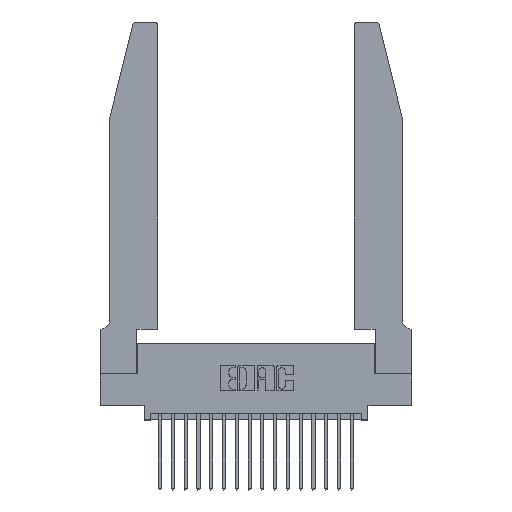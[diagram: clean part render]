
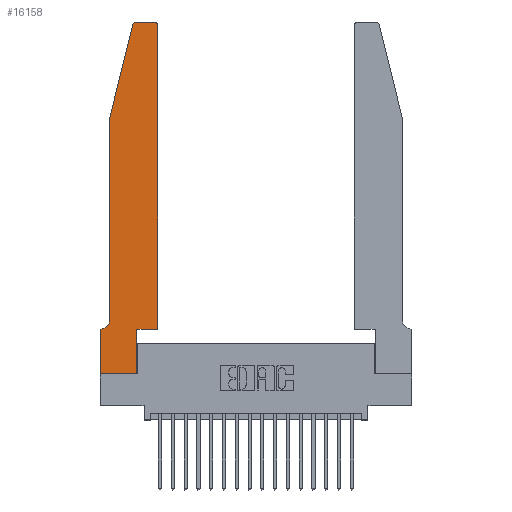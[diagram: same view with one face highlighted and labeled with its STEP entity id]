
A CAD part, top view. The second image highlights one B-rep face of the part: STEP entity #16158.
In plain terms, the highlighted planar face has unit normal (0, 0, 1).
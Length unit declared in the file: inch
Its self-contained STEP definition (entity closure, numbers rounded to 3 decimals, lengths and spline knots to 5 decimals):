
#399 = AXIS2_PLACEMENT_3D ( 'NONE', #18051, #5147, #11506 ) ;
#463 = VERTEX_POINT ( 'NONE', #5191 ) ;
#599 = CARTESIAN_POINT ( 'NONE',  ( 0.4205, 2.75, 0.37 ) ) ;
#695 = CARTESIAN_POINT ( 'NONE',  ( 0.4505, 0.35, 0.37 ) ) ;
#801 = DIRECTION ( 'NONE',  ( 1., 0., 0. ) ) ;
#951 = CARTESIAN_POINT ( 'NONE',  ( 0.0755, 2., 0.37 ) ) ;
#1317 = ORIENTED_EDGE ( 'NONE', *, *, #19890, .T. ) ;
#1614 = DIRECTION ( 'NONE',  ( 0., 0., -1. ) ) ;
#2020 = VECTOR ( 'NONE', #10911, 39.37008 ) ;
#2176 = VECTOR ( 'NONE', #19699, 39.37008 ) ;
#2252 = CARTESIAN_POINT ( 'NONE',  ( 0.4505, 0.35, 0.37 ) ) ;
#2361 = EDGE_CURVE ( 'NONE', #13977, #12685, #13348, .T. ) ;
#2386 = LINE ( 'NONE', #2812, #5926 ) ;
#2626 = DIRECTION ( 'NONE',  ( 1., 0., 0. ) ) ;
#2704 = EDGE_CURVE ( 'NONE', #16353, #9032, #15314, .T. ) ;
#2812 = CARTESIAN_POINT ( 'NONE',  ( 0.2605, 2.75, 0.37 ) ) ;
#2854 = CARTESIAN_POINT ( 'NONE',  ( 0.0755, 0.35, 0.37 ) ) ;
#2871 = DIRECTION ( 'NONE',  ( 0., 1., 0. ) ) ;
#3501 = CARTESIAN_POINT ( 'NONE',  ( 0., 0., 0.37 ) ) ;
#3580 = VERTEX_POINT ( 'NONE', #14657 ) ;
#3738 = VECTOR ( 'NONE', #4488, 39.37008 ) ;
#4261 = AXIS2_PLACEMENT_3D ( 'NONE', #4672, #1614, #6376 ) ;
#4352 = EDGE_CURVE ( 'NONE', #8377, #16353, #8440, .T. ) ;
#4411 = CARTESIAN_POINT ( 'NONE',  ( 0., 0.35, 0.37 ) ) ;
#4488 = DIRECTION ( 'NONE',  ( -1., 0., 0. ) ) ;
#4672 = CARTESIAN_POINT ( 'NONE',  ( 0.0055, 0.42, 0.37 ) ) ;
#5147 = DIRECTION ( 'NONE',  ( 0., 0., 1. ) ) ;
#5191 = CARTESIAN_POINT ( 'NONE',  ( 0.284, 2.75, 0.37 ) ) ;
#5315 = AXIS2_PLACEMENT_3D ( 'NONE', #18720, #5749, #2626 ) ;
#5669 = DIRECTION ( 'NONE',  ( -0.239, -0.971, 0. ) ) ;
#5749 = DIRECTION ( 'NONE',  ( 0., 0., 1. ) ) ;
#5926 = VECTOR ( 'NONE', #15539, 39.37008 ) ;
#6181 = VECTOR ( 'NONE', #13761, 39.37008 ) ;
#6376 = DIRECTION ( 'NONE',  ( -1., 0., 0. ) ) ;
#6508 = VECTOR ( 'NONE', #8860, 39.37008 ) ;
#6600 = LINE ( 'NONE', #7381, #2020 ) ;
#7084 = CARTESIAN_POINT ( 'NONE',  ( 0., 0.35, 0.37 ) ) ;
#7381 = CARTESIAN_POINT ( 'NONE',  ( 0., 0., 0.37 ) ) ;
#7890 = ORIENTED_EDGE ( 'NONE', *, *, #12336, .T. ) ;
#8083 = VECTOR ( 'NONE', #8981, 39.37008 ) ;
#8175 = ORIENTED_EDGE ( 'NONE', *, *, #2361, .T. ) ;
#8377 = VERTEX_POINT ( 'NONE', #20399 ) ;
#8440 = LINE ( 'NONE', #10752, #13260 ) ;
#8860 = DIRECTION ( 'NONE',  ( 1., 0., 0. ) ) ;
#8980 = CARTESIAN_POINT ( 'NONE',  ( 0.0055, 0.35, 0.37 ) ) ;
#8981 = DIRECTION ( 'NONE',  ( 0., 1., 0. ) ) ;
#9021 = CIRCLE ( 'NONE', #5315, 0.03 ) ;
#9032 = VERTEX_POINT ( 'NONE', #11317 ) ;
#9052 = ORIENTED_EDGE ( 'NONE', *, *, #17228, .T. ) ;
#9100 = CARTESIAN_POINT ( 'NONE',  ( 0.2865, 0.35, 0.37 ) ) ;
#9245 = EDGE_CURVE ( 'NONE', #3580, #11007, #9021, .T. ) ;
#9321 = CARTESIAN_POINT ( 'NONE',  ( 0., 0., 0.37 ) ) ;
#10720 = EDGE_CURVE ( 'NONE', #20834, #15609, #16432, .T. ) ;
#10752 = CARTESIAN_POINT ( 'NONE',  ( 0.2865, 0.35, 0.37 ) ) ;
#10911 = DIRECTION ( 'NONE',  ( 0., -1., 0. ) ) ;
#11007 = VERTEX_POINT ( 'NONE', #599 ) ;
#11317 = CARTESIAN_POINT ( 'NONE',  ( 0.4505, 0.35, 0.37 ) ) ;
#11506 = DIRECTION ( 'NONE',  ( 1., 0., 0. ) ) ;
#12031 = ORIENTED_EDGE ( 'NONE', *, *, #18009, .T. ) ;
#12162 = VECTOR ( 'NONE', #5669, 39.37008 ) ;
#12336 = EDGE_CURVE ( 'NONE', #12685, #16245, #12369, .T. ) ;
#12369 = LINE ( 'NONE', #2854, #3738 ) ;
#12685 = VERTEX_POINT ( 'NONE', #8980 ) ;
#12817 = VERTEX_POINT ( 'NONE', #9321 ) ;
#13169 = ORIENTED_EDGE ( 'NONE', *, *, #18387, .T. ) ;
#13260 = VECTOR ( 'NONE', #2871, 39.37008 ) ;
#13348 = CIRCLE ( 'NONE', #4261, 0.07 ) ;
#13761 = DIRECTION ( 'NONE',  ( 0., -1., 0. ) ) ;
#13977 = VERTEX_POINT ( 'NONE', #15450 ) ;
#14066 = EDGE_LOOP ( 'NONE', ( #17478, #1317, #17161, #9052, #8175, #7890, #12031, #16638, #20420, #14865, #13169, #17650 ) ) ;
#14475 = EDGE_CURVE ( 'NONE', #11007, #463, #2386, .T. ) ;
#14557 = CIRCLE ( 'NONE', #399, 0.03 ) ;
#14657 = CARTESIAN_POINT ( 'NONE',  ( 0.4505, 2.72, 0.37 ) ) ;
#14865 = ORIENTED_EDGE ( 'NONE', *, *, #2704, .T. ) ;
#15095 = PLANE ( 'NONE',  #16609 ) ;
#15314 = LINE ( 'NONE', #695, #6508 ) ;
#15329 = CARTESIAN_POINT ( 'NONE',  ( 0.0755, 2., 0.37 ) ) ;
#15343 = CARTESIAN_POINT ( 'NONE',  ( 0.0755, 2., 0.37 ) ) ;
#15450 = CARTESIAN_POINT ( 'NONE',  ( 0.0755, 0.42, 0.37 ) ) ;
#15490 = FACE_OUTER_BOUND ( 'NONE', #14066, .T. ) ;
#15539 = DIRECTION ( 'NONE',  ( -1., 0., 0. ) ) ;
#15609 = VERTEX_POINT ( 'NONE', #15343 ) ;
#15693 = CARTESIAN_POINT ( 'NONE',  ( 0.25487, 2.72718, 0.37 ) ) ;
#16158 = ADVANCED_FACE ( 'NONE', ( #15490 ), #15095, .T. ) ;
#16245 = VERTEX_POINT ( 'NONE', #4411 ) ;
#16353 = VERTEX_POINT ( 'NONE', #9100 ) ;
#16432 = LINE ( 'NONE', #15329, #12162 ) ;
#16609 = AXIS2_PLACEMENT_3D ( 'NONE', #7084, #16837, #801 ) ;
#16638 = ORIENTED_EDGE ( 'NONE', *, *, #19851, .T. ) ;
#16837 = DIRECTION ( 'NONE',  ( 0., 0., 1. ) ) ;
#17081 = LINE ( 'NONE', #3501, #2176 ) ;
#17161 = ORIENTED_EDGE ( 'NONE', *, *, #10720, .T. ) ;
#17228 = EDGE_CURVE ( 'NONE', #15609, #13977, #17266, .T. ) ;
#17266 = LINE ( 'NONE', #951, #6181 ) ;
#17478 = ORIENTED_EDGE ( 'NONE', *, *, #14475, .T. ) ;
#17650 = ORIENTED_EDGE ( 'NONE', *, *, #9245, .T. ) ;
#18009 = EDGE_CURVE ( 'NONE', #16245, #12817, #6600, .T. ) ;
#18051 = CARTESIAN_POINT ( 'NONE',  ( 0.284, 2.72, 0.37 ) ) ;
#18387 = EDGE_CURVE ( 'NONE', #9032, #3580, #20971, .T. ) ;
#18720 = CARTESIAN_POINT ( 'NONE',  ( 0.4205, 2.72, 0.37 ) ) ;
#19699 = DIRECTION ( 'NONE',  ( 1., 0., 0. ) ) ;
#19851 = EDGE_CURVE ( 'NONE', #12817, #8377, #17081, .T. ) ;
#19890 = EDGE_CURVE ( 'NONE', #463, #20834, #14557, .T. ) ;
#20399 = CARTESIAN_POINT ( 'NONE',  ( 0.2865, 0., 0.37 ) ) ;
#20420 = ORIENTED_EDGE ( 'NONE', *, *, #4352, .T. ) ;
#20834 = VERTEX_POINT ( 'NONE', #15693 ) ;
#20971 = LINE ( 'NONE', #2252, #8083 ) ;
